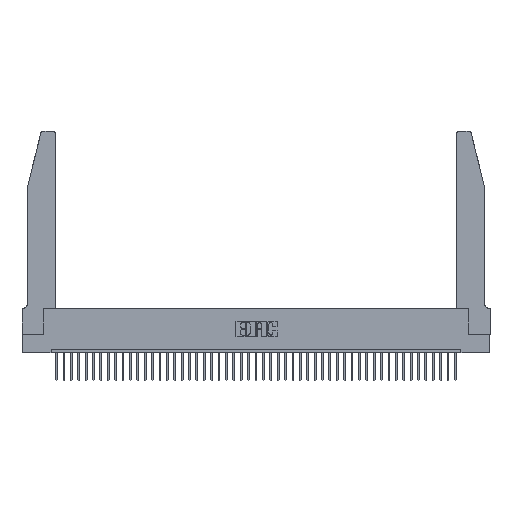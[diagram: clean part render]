
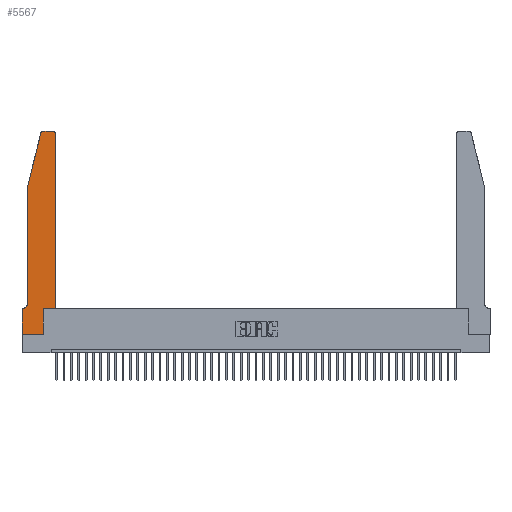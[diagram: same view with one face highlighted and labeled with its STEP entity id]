
A CAD part, top view. The second image highlights one B-rep face of the part: STEP entity #5567.
In plain terms, the highlighted planar face has unit normal (0, 0, 1).
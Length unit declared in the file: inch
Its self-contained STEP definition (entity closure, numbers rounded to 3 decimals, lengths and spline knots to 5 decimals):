
#165 = EDGE_CURVE ( 'NONE', #20931, #11257, #4580, .T. ) ;
#629 = AXIS2_PLACEMENT_3D ( 'NONE', #14436, #28059, #10863 ) ;
#1772 = LINE ( 'NONE', #42944, #41476 ) ;
#2954 = CARTESIAN_POINT ( 'NONE',  ( 0.0755, 2., 0.37 ) ) ;
#4580 = CIRCLE ( 'NONE', #629, 0.03 ) ;
#4822 = CARTESIAN_POINT ( 'NONE',  ( 0.4205, 2.75, 0.37 ) ) ;
#4880 = EDGE_CURVE ( 'NONE', #23662, #6762, #22186, .T. ) ;
#5212 = EDGE_CURVE ( 'NONE', #36543, #29170, #23825, .T. ) ;
#5395 = ORIENTED_EDGE ( 'NONE', *, *, #14319, .T. ) ;
#5567 = ADVANCED_FACE ( 'NONE', ( #27491 ), #20097, .T. ) ;
#5787 = DIRECTION ( 'NONE',  ( 0., 0., 1. ) ) ;
#6098 = DIRECTION ( 'NONE',  ( 1., 0., 0. ) ) ;
#6453 = CARTESIAN_POINT ( 'NONE',  ( 0., 0.35, 0.37 ) ) ;
#6648 = ORIENTED_EDGE ( 'NONE', *, *, #4880, .T. ) ;
#6762 = VERTEX_POINT ( 'NONE', #4822 ) ;
#6804 = AXIS2_PLACEMENT_3D ( 'NONE', #10544, #20572, #27738 ) ;
#7208 = CARTESIAN_POINT ( 'NONE',  ( 0.4505, 0.35, 0.37 ) ) ;
#7234 = CARTESIAN_POINT ( 'NONE',  ( 0.4505, 2.72, 0.37 ) ) ;
#7709 = LINE ( 'NONE', #2954, #10420 ) ;
#7876 = VECTOR ( 'NONE', #36316, 39.37008 ) ;
#7897 = CARTESIAN_POINT ( 'NONE',  ( 0., 0., 0.37 ) ) ;
#8674 = ORIENTED_EDGE ( 'NONE', *, *, #31459, .T. ) ;
#8864 = CARTESIAN_POINT ( 'NONE',  ( 0.0755, 0.42, 0.37 ) ) ;
#9415 = CARTESIAN_POINT ( 'NONE',  ( 0., 0., 0.37 ) ) ;
#9467 = CIRCLE ( 'NONE', #6804, 0.07 ) ;
#10089 = LINE ( 'NONE', #43170, #7876 ) ;
#10316 = DIRECTION ( 'NONE',  ( -0.239, -0.971, 0. ) ) ;
#10420 = VECTOR ( 'NONE', #10316, 39.37008 ) ;
#10478 = VECTOR ( 'NONE', #38255, 39.37008 ) ;
#10544 = CARTESIAN_POINT ( 'NONE',  ( 0.0055, 0.42, 0.37 ) ) ;
#10863 = DIRECTION ( 'NONE',  ( 1., 0., 0. ) ) ;
#11257 = VERTEX_POINT ( 'NONE', #28740 ) ;
#11722 = AXIS2_PLACEMENT_3D ( 'NONE', #12994, #33800, #36980 ) ;
#12171 = CARTESIAN_POINT ( 'NONE',  ( 0., 0., 0.37 ) ) ;
#12451 = CARTESIAN_POINT ( 'NONE',  ( 0.4505, 0.35, 0.37 ) ) ;
#12735 = ORIENTED_EDGE ( 'NONE', *, *, #35456, .T. ) ;
#12994 = CARTESIAN_POINT ( 'NONE',  ( 0.4205, 2.72, 0.37 ) ) ;
#13330 = ORIENTED_EDGE ( 'NONE', *, *, #29120, .T. ) ;
#13445 = VERTEX_POINT ( 'NONE', #30099 ) ;
#14226 = ORIENTED_EDGE ( 'NONE', *, *, #5212, .T. ) ;
#14230 = EDGE_CURVE ( 'NONE', #19179, #33837, #36904, .T. ) ;
#14319 = EDGE_CURVE ( 'NONE', #6762, #20931, #10089, .T. ) ;
#14436 = CARTESIAN_POINT ( 'NONE',  ( 0.284, 2.72, 0.37 ) ) ;
#15165 = ORIENTED_EDGE ( 'NONE', *, *, #165, .T. ) ;
#15213 = VECTOR ( 'NONE', #31423, 39.37008 ) ;
#15890 = DIRECTION ( 'NONE',  ( 1., 0., 0. ) ) ;
#17385 = CARTESIAN_POINT ( 'NONE',  ( 0.0755, 2., 0.37 ) ) ;
#18733 = EDGE_CURVE ( 'NONE', #29170, #13445, #23896, .T. ) ;
#19179 = VERTEX_POINT ( 'NONE', #21607 ) ;
#19808 = EDGE_CURVE ( 'NONE', #37983, #40304, #20612, .T. ) ;
#20097 = PLANE ( 'NONE',  #29502 ) ;
#20572 = DIRECTION ( 'NONE',  ( 0., 0., -1. ) ) ;
#20612 = LINE ( 'NONE', #38073, #15213 ) ;
#20931 = VERTEX_POINT ( 'NONE', #43585 ) ;
#21583 = ORIENTED_EDGE ( 'NONE', *, *, #42173, .T. ) ;
#21607 = CARTESIAN_POINT ( 'NONE',  ( 0.0055, 0.35, 0.37 ) ) ;
#22186 = CIRCLE ( 'NONE', #11722, 0.03 ) ;
#23662 = VERTEX_POINT ( 'NONE', #7234 ) ;
#23825 = LINE ( 'NONE', #9415, #32302 ) ;
#23896 = LINE ( 'NONE', #42187, #10478 ) ;
#24601 = LINE ( 'NONE', #12451, #32598 ) ;
#26521 = CARTESIAN_POINT ( 'NONE',  ( 0.0755, 0.35, 0.37 ) ) ;
#27491 = FACE_OUTER_BOUND ( 'NONE', #38150, .T. ) ;
#27516 = VERTEX_POINT ( 'NONE', #7208 ) ;
#27738 = DIRECTION ( 'NONE',  ( -1., 0., 0. ) ) ;
#28059 = DIRECTION ( 'NONE',  ( 0., 0., 1. ) ) ;
#28435 = ORIENTED_EDGE ( 'NONE', *, *, #18733, .T. ) ;
#28688 = VECTOR ( 'NONE', #36160, 39.37008 ) ;
#28740 = CARTESIAN_POINT ( 'NONE',  ( 0.25487, 2.72718, 0.37 ) ) ;
#28796 = VECTOR ( 'NONE', #40451, 39.37008 ) ;
#29120 = EDGE_CURVE ( 'NONE', #40304, #19179, #9467, .T. ) ;
#29170 = VERTEX_POINT ( 'NONE', #31009 ) ;
#29502 = AXIS2_PLACEMENT_3D ( 'NONE', #6453, #5787, #41120 ) ;
#30099 = CARTESIAN_POINT ( 'NONE',  ( 0.2865, 0.35, 0.37 ) ) ;
#31009 = CARTESIAN_POINT ( 'NONE',  ( 0.2865, 0., 0.37 ) ) ;
#31423 = DIRECTION ( 'NONE',  ( 0., -1., 0. ) ) ;
#31459 = EDGE_CURVE ( 'NONE', #27516, #23662, #1772, .T. ) ;
#32302 = VECTOR ( 'NONE', #6098, 39.37008 ) ;
#32440 = DIRECTION ( 'NONE',  ( 0., 1., 0. ) ) ;
#32598 = VECTOR ( 'NONE', #15890, 39.37008 ) ;
#33800 = DIRECTION ( 'NONE',  ( 0., 0., 1. ) ) ;
#33837 = VERTEX_POINT ( 'NONE', #41028 ) ;
#35456 = EDGE_CURVE ( 'NONE', #13445, #27516, #24601, .T. ) ;
#36160 = DIRECTION ( 'NONE',  ( 0., -1., 0. ) ) ;
#36316 = DIRECTION ( 'NONE',  ( -1., 0., 0. ) ) ;
#36543 = VERTEX_POINT ( 'NONE', #7897 ) ;
#36770 = ORIENTED_EDGE ( 'NONE', *, *, #19808, .T. ) ;
#36904 = LINE ( 'NONE', #26521, #28796 ) ;
#36980 = DIRECTION ( 'NONE',  ( 1., 0., 0. ) ) ;
#37198 = ORIENTED_EDGE ( 'NONE', *, *, #14230, .T. ) ;
#37983 = VERTEX_POINT ( 'NONE', #17385 ) ;
#38073 = CARTESIAN_POINT ( 'NONE',  ( 0.0755, 2., 0.37 ) ) ;
#38150 = EDGE_LOOP ( 'NONE', ( #5395, #15165, #38517, #36770, #13330, #37198, #21583, #14226, #28435, #12735, #8674, #6648 ) ) ;
#38255 = DIRECTION ( 'NONE',  ( 0., 1., 0. ) ) ;
#38517 = ORIENTED_EDGE ( 'NONE', *, *, #38564, .T. ) ;
#38564 = EDGE_CURVE ( 'NONE', #11257, #37983, #7709, .T. ) ;
#40304 = VERTEX_POINT ( 'NONE', #8864 ) ;
#40451 = DIRECTION ( 'NONE',  ( -1., 0., 0. ) ) ;
#41028 = CARTESIAN_POINT ( 'NONE',  ( 0., 0.35, 0.37 ) ) ;
#41120 = DIRECTION ( 'NONE',  ( 1., 0., 0. ) ) ;
#41476 = VECTOR ( 'NONE', #32440, 39.37008 ) ;
#42173 = EDGE_CURVE ( 'NONE', #33837, #36543, #43712, .T. ) ;
#42187 = CARTESIAN_POINT ( 'NONE',  ( 0.2865, 0.35, 0.37 ) ) ;
#42944 = CARTESIAN_POINT ( 'NONE',  ( 0.4505, 0.35, 0.37 ) ) ;
#43170 = CARTESIAN_POINT ( 'NONE',  ( 0.2605, 2.75, 0.37 ) ) ;
#43585 = CARTESIAN_POINT ( 'NONE',  ( 0.284, 2.75, 0.37 ) ) ;
#43712 = LINE ( 'NONE', #12171, #28688 ) ;
